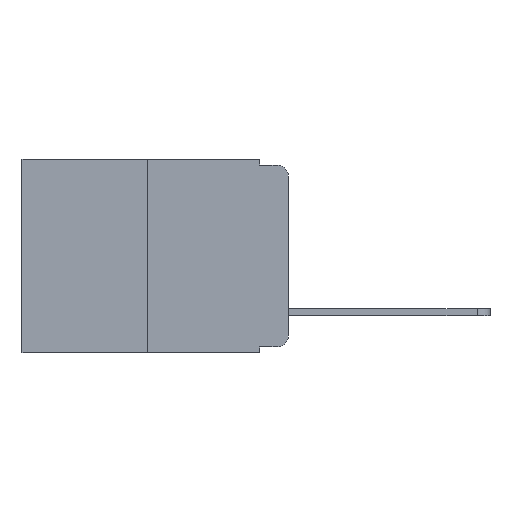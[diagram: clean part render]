
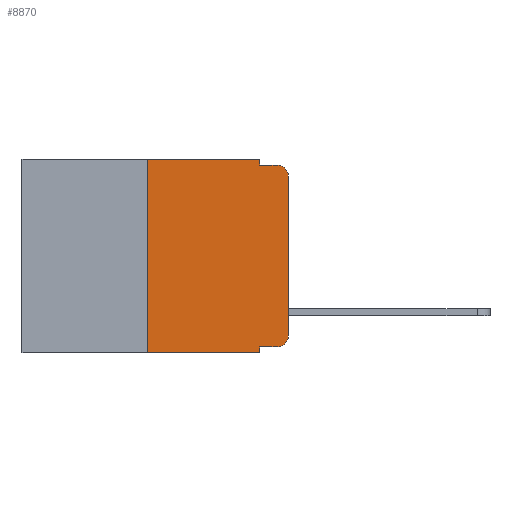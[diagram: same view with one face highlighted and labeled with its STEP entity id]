
A CAD part, left-side view. The second image highlights one B-rep face of the part: STEP entity #8870.
In plain terms, the highlighted planar face has unit normal (-1, 0, 0).
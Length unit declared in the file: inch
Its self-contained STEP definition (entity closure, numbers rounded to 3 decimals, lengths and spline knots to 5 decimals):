
#75 = DIRECTION ( 'NONE',  ( 0., 0., -1. ) ) ;
#161 = EDGE_CURVE ( 'NONE', #2149, #9264, #9128, .T. ) ;
#509 = CARTESIAN_POINT ( 'NONE',  ( 0., 0., 0. ) ) ;
#609 = CARTESIAN_POINT ( 'NONE',  ( 0., 0.25, 0. ) ) ;
#656 = DIRECTION ( 'NONE',  ( 0., 0., 1. ) ) ;
#839 = ORIENTED_EDGE ( 'NONE', *, *, #2091, .F. ) ;
#903 = ORIENTED_EDGE ( 'NONE', *, *, #4280, .F. ) ;
#1025 = ORIENTED_EDGE ( 'NONE', *, *, #7289, .F. ) ;
#1045 = VECTOR ( 'NONE', #9040, 39.37008 ) ;
#1413 = CARTESIAN_POINT ( 'NONE',  ( 0., 0.051, 0. ) ) ;
#1449 = DIRECTION ( 'NONE',  ( 0., -1., 0. ) ) ;
#1565 = ORIENTED_EDGE ( 'NONE', *, *, #5211, .T. ) ;
#1629 = DIRECTION ( 'NONE',  ( 0., 0., -1. ) ) ;
#1786 = VERTEX_POINT ( 'NONE', #5329 ) ;
#1815 = ORIENTED_EDGE ( 'NONE', *, *, #161, .F. ) ;
#1873 = DIRECTION ( 'NONE',  ( 0., -1., 0. ) ) ;
#2091 = EDGE_CURVE ( 'NONE', #2937, #5763, #4225, .T. ) ;
#2095 = CARTESIAN_POINT ( 'NONE',  ( 0., 0.02, -0.03 ) ) ;
#2106 = VECTOR ( 'NONE', #1449, 39.37008 ) ;
#2144 = DIRECTION ( 'NONE',  ( -1., 0., 0. ) ) ;
#2149 = VERTEX_POINT ( 'NONE', #9526 ) ;
#2218 = CARTESIAN_POINT ( 'NONE',  ( 0., 0.051, 0. ) ) ;
#2451 = DIRECTION ( 'NONE',  ( 1., 0., 0. ) ) ;
#2506 = VERTEX_POINT ( 'NONE', #9576 ) ;
#2524 = LINE ( 'NONE', #1413, #8168 ) ;
#2574 = CIRCLE ( 'NONE', #7702, 0.02 ) ;
#2817 = AXIS2_PLACEMENT_3D ( 'NONE', #2095, #2144, #75 ) ;
#2937 = VERTEX_POINT ( 'NONE', #5824 ) ;
#2973 = VERTEX_POINT ( 'NONE', #4842 ) ;
#3014 = DIRECTION ( 'NONE',  ( 0., 0., -1. ) ) ;
#3082 = DIRECTION ( 'NONE',  ( -1., 0., 0. ) ) ;
#3177 = CARTESIAN_POINT ( 'NONE',  ( 0., 0.02, -0.313 ) ) ;
#3258 = EDGE_CURVE ( 'NONE', #2973, #2149, #3587, .T. ) ;
#3381 = EDGE_CURVE ( 'NONE', #6166, #1786, #2574, .T. ) ;
#3534 = VERTEX_POINT ( 'NONE', #5765 ) ;
#3587 = LINE ( 'NONE', #609, #5468 ) ;
#3739 = CARTESIAN_POINT ( 'NONE',  ( 0., 0.473, 0. ) ) ;
#3778 = CARTESIAN_POINT ( 'NONE',  ( 0., 0.051, -0.333 ) ) ;
#3817 = DIRECTION ( 'NONE',  ( 0., 0., -1. ) ) ;
#3826 = LINE ( 'NONE', #2218, #9924 ) ;
#3961 = CARTESIAN_POINT ( 'NONE',  ( 0., 0.051, 0. ) ) ;
#4029 = ORIENTED_EDGE ( 'NONE', *, *, #9437, .T. ) ;
#4221 = VECTOR ( 'NONE', #1873, 39.37008 ) ;
#4225 = LINE ( 'NONE', #9920, #2106 ) ;
#4280 = EDGE_CURVE ( 'NONE', #5030, #3534, #3826, .T. ) ;
#4446 = EDGE_LOOP ( 'NONE', ( #6586, #4596, #839, #1025, #1815, #5885, #1565, #903, #4029, #4685 ) ) ;
#4596 = ORIENTED_EDGE ( 'NONE', *, *, #5025, .T. ) ;
#4685 = ORIENTED_EDGE ( 'NONE', *, *, #3381, .T. ) ;
#4842 = CARTESIAN_POINT ( 'NONE',  ( 0., 0.25, -0.343 ) ) ;
#5025 = EDGE_CURVE ( 'NONE', #2506, #5763, #8674, .T. ) ;
#5030 = VERTEX_POINT ( 'NONE', #3778 ) ;
#5211 = EDGE_CURVE ( 'NONE', #2973, #3534, #8549, .T. ) ;
#5323 = DIRECTION ( 'NONE',  ( 0., -1., 0. ) ) ;
#5329 = CARTESIAN_POINT ( 'NONE',  ( 0., 0., -0.313 ) ) ;
#5386 = CARTESIAN_POINT ( 'NONE',  ( 0., 0.02, -0.333 ) ) ;
#5394 = VECTOR ( 'NONE', #5323, 39.37008 ) ;
#5468 = VECTOR ( 'NONE', #656, 39.37008 ) ;
#5580 = CARTESIAN_POINT ( 'NONE',  ( 0., 0.02, -0.01 ) ) ;
#5763 = VERTEX_POINT ( 'NONE', #5580 ) ;
#5765 = CARTESIAN_POINT ( 'NONE',  ( 0., 0.051, -0.343 ) ) ;
#5824 = CARTESIAN_POINT ( 'NONE',  ( 0., 0.051, -0.01 ) ) ;
#5885 = ORIENTED_EDGE ( 'NONE', *, *, #3258, .F. ) ;
#5925 = VECTOR ( 'NONE', #8259, 39.37008 ) ;
#6166 = VERTEX_POINT ( 'NONE', #5386 ) ;
#6379 = PLANE ( 'NONE',  #7458 ) ;
#6491 = LINE ( 'NONE', #7243, #4221 ) ;
#6586 = ORIENTED_EDGE ( 'NONE', *, *, #10138, .T. ) ;
#7079 = CARTESIAN_POINT ( 'NONE',  ( 0., 0.473, 0. ) ) ;
#7243 = CARTESIAN_POINT ( 'NONE',  ( 0., 0.051, -0.333 ) ) ;
#7289 = EDGE_CURVE ( 'NONE', #9264, #2937, #2524, .T. ) ;
#7458 = AXIS2_PLACEMENT_3D ( 'NONE', #7079, #2451, #7844 ) ;
#7702 = AXIS2_PLACEMENT_3D ( 'NONE', #3177, #3082, #3014 ) ;
#7844 = DIRECTION ( 'NONE',  ( 0., 0., -1. ) ) ;
#8100 = LINE ( 'NONE', #509, #5925 ) ;
#8168 = VECTOR ( 'NONE', #3817, 39.37008 ) ;
#8259 = DIRECTION ( 'NONE',  ( 0., 0., 1. ) ) ;
#8549 = LINE ( 'NONE', #8619, #1045 ) ;
#8619 = CARTESIAN_POINT ( 'NONE',  ( 0., 0.473, -0.343 ) ) ;
#8674 = CIRCLE ( 'NONE', #2817, 0.02 ) ;
#8870 = ADVANCED_FACE ( 'NONE', ( #9348 ), #6379, .F. ) ;
#9040 = DIRECTION ( 'NONE',  ( 0., -1., 0. ) ) ;
#9128 = LINE ( 'NONE', #3739, #5394 ) ;
#9264 = VERTEX_POINT ( 'NONE', #3961 ) ;
#9348 = FACE_OUTER_BOUND ( 'NONE', #4446, .T. ) ;
#9437 = EDGE_CURVE ( 'NONE', #5030, #6166, #6491, .T. ) ;
#9526 = CARTESIAN_POINT ( 'NONE',  ( 0., 0.25, 0. ) ) ;
#9576 = CARTESIAN_POINT ( 'NONE',  ( 0., 0., -0.03 ) ) ;
#9920 = CARTESIAN_POINT ( 'NONE',  ( 0., 0.051, -0.01 ) ) ;
#9924 = VECTOR ( 'NONE', #1629, 39.37008 ) ;
#10138 = EDGE_CURVE ( 'NONE', #1786, #2506, #8100, .T. ) ;
